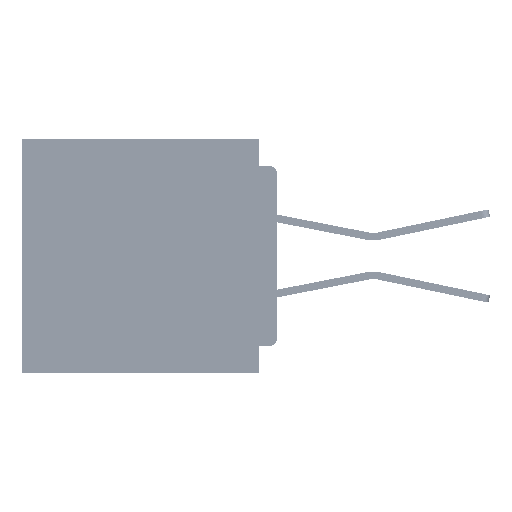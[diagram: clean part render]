
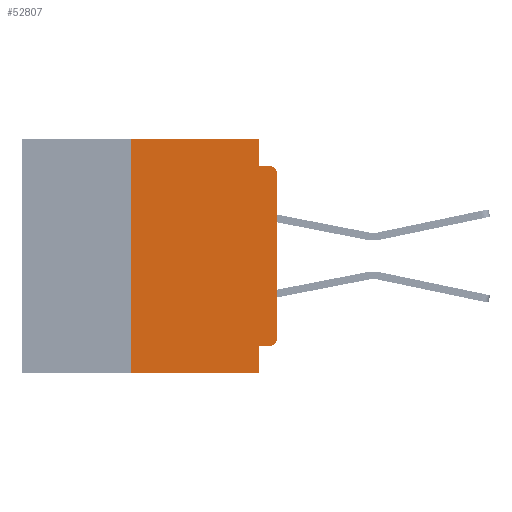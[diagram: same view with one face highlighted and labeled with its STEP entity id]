
A CAD part, left-side view. The second image highlights one B-rep face of the part: STEP entity #52807.
In plain terms, the highlighted planar face has unit normal (-1, 0, 0).
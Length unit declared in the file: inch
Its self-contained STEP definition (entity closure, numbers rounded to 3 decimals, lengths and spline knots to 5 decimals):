
#657 = ORIENTED_EDGE ( 'NONE', *, *, #26885, .T. ) ;
#793 = DIRECTION ( 'NONE',  ( 0., 0., -1. ) ) ;
#2098 = VECTOR ( 'NONE', #6098, 39.37008 ) ;
#2836 = ORIENTED_EDGE ( 'NONE', *, *, #65405, .F. ) ;
#2983 = AXIS2_PLACEMENT_3D ( 'NONE', #67586, #35561, #3538 ) ;
#3538 = DIRECTION ( 'NONE',  ( 0., 0., -1. ) ) ;
#4027 = DIRECTION ( 'NONE',  ( 0., -1., 0. ) ) ;
#5221 = CIRCLE ( 'NONE', #2983, 0.015 ) ;
#6098 = DIRECTION ( 'NONE',  ( 0., -1., 0. ) ) ;
#7450 = CARTESIAN_POINT ( 'NONE',  ( 0., 0.437, 0. ) ) ;
#7978 = CARTESIAN_POINT ( 'NONE',  ( 0., 0.031, -0.4 ) ) ;
#8301 = AXIS2_PLACEMENT_3D ( 'NONE', #64840, #32771, #793 ) ;
#8457 = DIRECTION ( 'NONE',  ( 0., 0., 1. ) ) ;
#8741 = LINE ( 'NONE', #7978, #63927 ) ;
#9210 = VERTEX_POINT ( 'NONE', #17788 ) ;
#10360 = VERTEX_POINT ( 'NONE', #23742 ) ;
#11727 = EDGE_LOOP ( 'NONE', ( #40790, #657, #63464, #17805, #2836, #49586, #16638, #30207, #33994, #58105 ) ) ;
#11959 = VERTEX_POINT ( 'NONE', #58400 ) ;
#13467 = CARTESIAN_POINT ( 'NONE',  ( 0., 0.015, -0.34 ) ) ;
#16306 = CARTESIAN_POINT ( 'NONE',  ( 0., 0., -0.355 ) ) ;
#16629 = LINE ( 'NONE', #7450, #55905 ) ;
#16638 = ORIENTED_EDGE ( 'NONE', *, *, #50287, .T. ) ;
#17788 = CARTESIAN_POINT ( 'NONE',  ( 0., 0.25, -0.4 ) ) ;
#17805 = ORIENTED_EDGE ( 'NONE', *, *, #49168, .F. ) ;
#17945 = DIRECTION ( 'NONE',  ( 0., 0., 1. ) ) ;
#18824 = DIRECTION ( 'NONE',  ( 0., 0., -1. ) ) ;
#23200 = VERTEX_POINT ( 'NONE', #56324 ) ;
#23742 = CARTESIAN_POINT ( 'NONE',  ( 0., 0.031, -0.4 ) ) ;
#25487 = VECTOR ( 'NONE', #17945, 39.37008 ) ;
#26782 = DIRECTION ( 'NONE',  ( 0., 1., 0. ) ) ;
#26885 = EDGE_CURVE ( 'NONE', #41736, #11959, #5221, .T. ) ;
#26907 = FACE_OUTER_BOUND ( 'NONE', #11727, .T. ) ;
#30051 = CARTESIAN_POINT ( 'NONE',  ( 0., 0.031, -0.355 ) ) ;
#30053 = VERTEX_POINT ( 'NONE', #30051 ) ;
#30207 = ORIENTED_EDGE ( 'NONE', *, *, #61232, .F. ) ;
#32160 = LINE ( 'NONE', #32675, #2098 ) ;
#32675 = CARTESIAN_POINT ( 'NONE',  ( 0., 0.437, -0.4 ) ) ;
#32771 = DIRECTION ( 'NONE',  ( 1., 0., 0. ) ) ;
#33994 = ORIENTED_EDGE ( 'NONE', *, *, #39416, .F. ) ;
#34484 = CARTESIAN_POINT ( 'NONE',  ( 0., 0.25, 0. ) ) ;
#35082 = CARTESIAN_POINT ( 'NONE',  ( 0., 0.25, -0.4 ) ) ;
#35561 = DIRECTION ( 'NONE',  ( -1., 0., 0. ) ) ;
#38897 = LINE ( 'NONE', #68063, #65604 ) ;
#39207 = CARTESIAN_POINT ( 'NONE',  ( 0., 0.031, 0. ) ) ;
#39416 = EDGE_CURVE ( 'NONE', #44044, #30053, #47195, .T. ) ;
#39741 = LINE ( 'NONE', #65839, #25487 ) ;
#40790 = ORIENTED_EDGE ( 'NONE', *, *, #67270, .T. ) ;
#41258 = CARTESIAN_POINT ( 'NONE',  ( 0., 0.015, -0.355 ) ) ;
#41736 = VERTEX_POINT ( 'NONE', #66273 ) ;
#44044 = VERTEX_POINT ( 'NONE', #41258 ) ;
#44590 = DIRECTION ( 'NONE',  ( 0., 0., -1. ) ) ;
#44872 = DIRECTION ( 'NONE',  ( 0., -1., 0. ) ) ;
#45768 = LINE ( 'NONE', #39207, #47436 ) ;
#45775 = EDGE_CURVE ( 'NONE', #9210, #59090, #56593, .T. ) ;
#47195 = LINE ( 'NONE', #16306, #59745 ) ;
#47436 = VECTOR ( 'NONE', #44590, 39.37008 ) ;
#48270 = CARTESIAN_POINT ( 'NONE',  ( 0., 0.031, 0. ) ) ;
#49168 = EDGE_CURVE ( 'NONE', #57662, #23200, #45768, .T. ) ;
#49586 = ORIENTED_EDGE ( 'NONE', *, *, #45775, .F. ) ;
#50287 = EDGE_CURVE ( 'NONE', #9210, #10360, #32160, .T. ) ;
#50855 = DIRECTION ( 'NONE',  ( -1., 0., 0. ) ) ;
#51074 = EDGE_CURVE ( 'NONE', #44044, #64980, #52279, .T. ) ;
#51302 = EDGE_CURVE ( 'NONE', #23200, #11959, #38897, .T. ) ;
#52279 = CIRCLE ( 'NONE', #57048, 0.015 ) ;
#52807 = ADVANCED_FACE ( 'NONE', ( #26907 ), #59476, .F. ) ;
#53248 = VECTOR ( 'NONE', #8457, 39.37008 ) ;
#55905 = VECTOR ( 'NONE', #44872, 39.37008 ) ;
#56137 = DIRECTION ( 'NONE',  ( 0., 0., -1. ) ) ;
#56324 = CARTESIAN_POINT ( 'NONE',  ( 0., 0.031, -0.045 ) ) ;
#56593 = LINE ( 'NONE', #35082, #53248 ) ;
#57048 = AXIS2_PLACEMENT_3D ( 'NONE', #13467, #50855, #18824 ) ;
#57305 = CARTESIAN_POINT ( 'NONE',  ( 0., 0., -0.34 ) ) ;
#57662 = VERTEX_POINT ( 'NONE', #48270 ) ;
#58105 = ORIENTED_EDGE ( 'NONE', *, *, #51074, .T. ) ;
#58400 = CARTESIAN_POINT ( 'NONE',  ( 0., 0.015, -0.045 ) ) ;
#59090 = VERTEX_POINT ( 'NONE', #34484 ) ;
#59476 = PLANE ( 'NONE',  #8301 ) ;
#59745 = VECTOR ( 'NONE', #26782, 39.37008 ) ;
#61232 = EDGE_CURVE ( 'NONE', #30053, #10360, #8741, .T. ) ;
#63464 = ORIENTED_EDGE ( 'NONE', *, *, #51302, .F. ) ;
#63927 = VECTOR ( 'NONE', #56137, 39.37008 ) ;
#64840 = CARTESIAN_POINT ( 'NONE',  ( 0., 0.437, 0. ) ) ;
#64980 = VERTEX_POINT ( 'NONE', #57305 ) ;
#65405 = EDGE_CURVE ( 'NONE', #59090, #57662, #16629, .T. ) ;
#65604 = VECTOR ( 'NONE', #4027, 39.37008 ) ;
#65839 = CARTESIAN_POINT ( 'NONE',  ( 0., 0., 0. ) ) ;
#66273 = CARTESIAN_POINT ( 'NONE',  ( 0., 0., -0.06 ) ) ;
#67270 = EDGE_CURVE ( 'NONE', #64980, #41736, #39741, .T. ) ;
#67586 = CARTESIAN_POINT ( 'NONE',  ( 0., 0.015, -0.06 ) ) ;
#68063 = CARTESIAN_POINT ( 'NONE',  ( 0., 0., -0.045 ) ) ;
